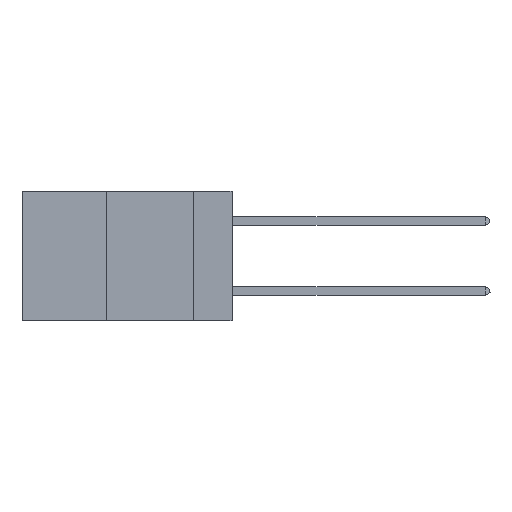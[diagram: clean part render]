
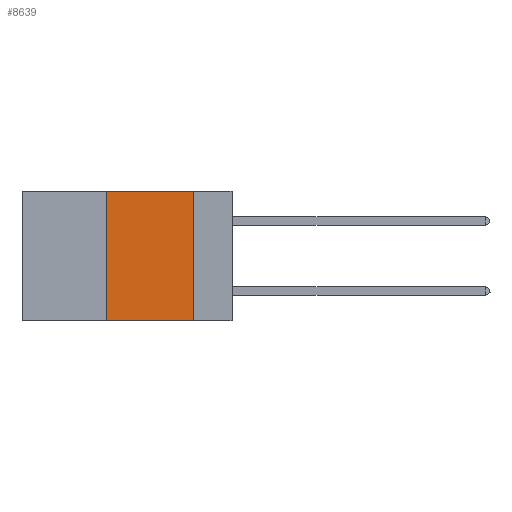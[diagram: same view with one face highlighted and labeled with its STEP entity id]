
A CAD part, left-side view. The second image highlights one B-rep face of the part: STEP entity #8639.
In plain terms, the highlighted planar face has unit normal (-1, 0, 0).
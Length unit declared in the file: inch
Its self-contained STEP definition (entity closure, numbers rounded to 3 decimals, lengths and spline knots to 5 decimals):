
#1124 = EDGE_CURVE ( 'NONE', #4619, #19938, #37757, .T. ) ;
#1275 = CARTESIAN_POINT ( 'NONE',  ( 0., 0.6, -0.37 ) ) ;
#1843 = LINE ( 'NONE', #41564, #40586 ) ;
#2211 = DIRECTION ( 'NONE',  ( 0., 0., 1. ) ) ;
#4619 = VERTEX_POINT ( 'NONE', #36788 ) ;
#7771 = CARTESIAN_POINT ( 'NONE',  ( 0., 0.6, 0. ) ) ;
#8342 = DIRECTION ( 'NONE',  ( 0., 0., -1. ) ) ;
#8639 = ADVANCED_FACE ( 'NONE', ( #34727 ), #18542, .F. ) ;
#9139 = VECTOR ( 'NONE', #2211, 39.37008 ) ;
#11662 = DIRECTION ( 'NONE',  ( 0., 0., -1. ) ) ;
#12669 = ORIENTED_EDGE ( 'NONE', *, *, #16745, .F. ) ;
#13670 = CARTESIAN_POINT ( 'NONE',  ( 0., 0.11, 0. ) ) ;
#14683 = DIRECTION ( 'NONE',  ( 0., -1., 0. ) ) ;
#16745 = EDGE_CURVE ( 'NONE', #34355, #19938, #1843, .T. ) ;
#17150 = ORIENTED_EDGE ( 'NONE', *, *, #42461, .F. ) ;
#18075 = LINE ( 'NONE', #18937, #40367 ) ;
#18542 = PLANE ( 'NONE',  #36725 ) ;
#18937 = CARTESIAN_POINT ( 'NONE',  ( 0., 0.6, 0. ) ) ;
#19938 = VERTEX_POINT ( 'NONE', #20535 ) ;
#20445 = VERTEX_POINT ( 'NONE', #27165 ) ;
#20535 = CARTESIAN_POINT ( 'NONE',  ( 0., 0.11, -0.37 ) ) ;
#22274 = LINE ( 'NONE', #28738, #9139 ) ;
#25010 = DIRECTION ( 'NONE',  ( 1., 0., 0. ) ) ;
#26629 = VECTOR ( 'NONE', #14683, 39.37008 ) ;
#27165 = CARTESIAN_POINT ( 'NONE',  ( 0., 0.36, 0. ) ) ;
#28201 = DIRECTION ( 'NONE',  ( 0., -1., 0. ) ) ;
#28712 = ORIENTED_EDGE ( 'NONE', *, *, #31735, .F. ) ;
#28738 = CARTESIAN_POINT ( 'NONE',  ( 0., 0.36, 0. ) ) ;
#30766 = EDGE_LOOP ( 'NONE', ( #12669, #28712, #17150, #40777 ) ) ;
#31735 = EDGE_CURVE ( 'NONE', #20445, #34355, #18075, .T. ) ;
#34355 = VERTEX_POINT ( 'NONE', #13670 ) ;
#34727 = FACE_OUTER_BOUND ( 'NONE', #30766, .T. ) ;
#36725 = AXIS2_PLACEMENT_3D ( 'NONE', #7771, #25010, #11662 ) ;
#36788 = CARTESIAN_POINT ( 'NONE',  ( 0., 0.36, -0.37 ) ) ;
#37757 = LINE ( 'NONE', #1275, #26629 ) ;
#40367 = VECTOR ( 'NONE', #28201, 39.37008 ) ;
#40586 = VECTOR ( 'NONE', #8342, 39.37008 ) ;
#40777 = ORIENTED_EDGE ( 'NONE', *, *, #1124, .T. ) ;
#41564 = CARTESIAN_POINT ( 'NONE',  ( 0., 0.11, 0. ) ) ;
#42461 = EDGE_CURVE ( 'NONE', #4619, #20445, #22274, .T. ) ;
